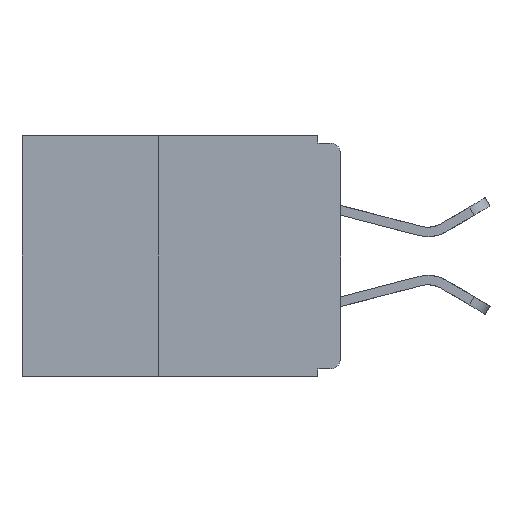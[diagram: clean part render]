
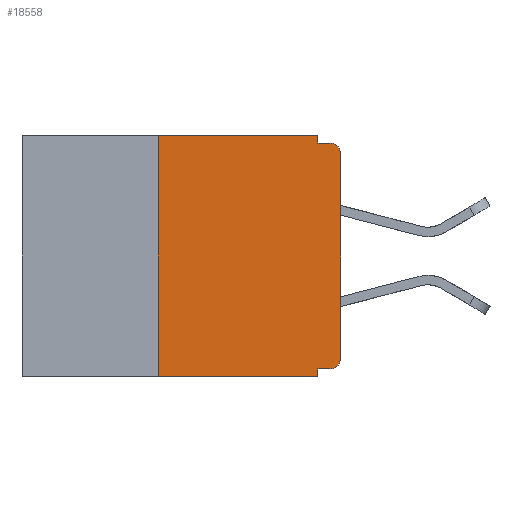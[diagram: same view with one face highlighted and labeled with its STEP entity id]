
A CAD part, left-side view. The second image highlights one B-rep face of the part: STEP entity #18558.
In plain terms, the highlighted planar face has unit normal (-1, 0, 0).
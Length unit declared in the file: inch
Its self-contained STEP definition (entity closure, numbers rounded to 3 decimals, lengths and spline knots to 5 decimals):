
#775 = ORIENTED_EDGE ( 'NONE', *, *, #17930, .F. ) ;
#1948 = CARTESIAN_POINT ( 'NONE',  ( 0., 0.25, -0.33 ) ) ;
#2475 = CARTESIAN_POINT ( 'NONE',  ( 0., 0.015, -0.01 ) ) ;
#2659 = CARTESIAN_POINT ( 'NONE',  ( 0., 0.031, 0. ) ) ;
#2809 = CARTESIAN_POINT ( 'NONE',  ( 0., 0.015, -0.025 ) ) ;
#2883 = DIRECTION ( 'NONE',  ( -1., 0., 0. ) ) ;
#2923 = CIRCLE ( 'NONE', #19588, 0.015 ) ;
#2995 = LINE ( 'NONE', #13170, #19923 ) ;
#3387 = LINE ( 'NONE', #9181, #15979 ) ;
#3621 = DIRECTION ( 'NONE',  ( 0., 0., 1. ) ) ;
#3716 = EDGE_CURVE ( 'NONE', #3820, #6808, #9754, .T. ) ;
#3820 = VERTEX_POINT ( 'NONE', #16730 ) ;
#4018 = CARTESIAN_POINT ( 'NONE',  ( 0., 0.437, -0.33 ) ) ;
#4341 = VECTOR ( 'NONE', #11575, 39.37008 ) ;
#4494 = DIRECTION ( 'NONE',  ( 0., 0., -1. ) ) ;
#4537 = VERTEX_POINT ( 'NONE', #20589 ) ;
#4973 = CIRCLE ( 'NONE', #15085, 0.015 ) ;
#4975 = VERTEX_POINT ( 'NONE', #13607 ) ;
#5214 = VERTEX_POINT ( 'NONE', #2659 ) ;
#5506 = AXIS2_PLACEMENT_3D ( 'NONE', #8097, #12951, #21109 ) ;
#5815 = VERTEX_POINT ( 'NONE', #5926 ) ;
#5926 = CARTESIAN_POINT ( 'NONE',  ( 0., 0.25, 0. ) ) ;
#6296 = EDGE_LOOP ( 'NONE', ( #6617, #12294, #13657, #19914, #775, #10690, #9777, #7531, #16128, #19337 ) ) ;
#6616 = CARTESIAN_POINT ( 'NONE',  ( 0., 0.015, -0.32 ) ) ;
#6617 = ORIENTED_EDGE ( 'NONE', *, *, #21088, .T. ) ;
#6808 = VERTEX_POINT ( 'NONE', #11500 ) ;
#7531 = ORIENTED_EDGE ( 'NONE', *, *, #3716, .F. ) ;
#7636 = LINE ( 'NONE', #16426, #20148 ) ;
#8097 = CARTESIAN_POINT ( 'NONE',  ( 0., 0.437, 0. ) ) ;
#8129 = DIRECTION ( 'NONE',  ( 0., -1., 0. ) ) ;
#8665 = VERTEX_POINT ( 'NONE', #13303 ) ;
#8786 = EDGE_CURVE ( 'NONE', #5214, #15198, #13096, .T. ) ;
#9181 = CARTESIAN_POINT ( 'NONE',  ( 0., 0., -0.01 ) ) ;
#9744 = PLANE ( 'NONE',  #5506 ) ;
#9754 = LINE ( 'NONE', #9954, #4341 ) ;
#9777 = ORIENTED_EDGE ( 'NONE', *, *, #13470, .T. ) ;
#9954 = CARTESIAN_POINT ( 'NONE',  ( 0., 0.031, -0.33 ) ) ;
#10346 = DIRECTION ( 'NONE',  ( 0., 0., -1. ) ) ;
#10690 = ORIENTED_EDGE ( 'NONE', *, *, #18111, .F. ) ;
#10864 = DIRECTION ( 'NONE',  ( 0., -1., 0. ) ) ;
#11077 = FACE_OUTER_BOUND ( 'NONE', #6296, .T. ) ;
#11475 = VERTEX_POINT ( 'NONE', #2475 ) ;
#11500 = CARTESIAN_POINT ( 'NONE',  ( 0., 0.031, -0.33 ) ) ;
#11575 = DIRECTION ( 'NONE',  ( 0., 0., -1. ) ) ;
#12294 = ORIENTED_EDGE ( 'NONE', *, *, #15626, .T. ) ;
#12762 = CARTESIAN_POINT ( 'NONE',  ( 0., 0.015, -0.305 ) ) ;
#12839 = CARTESIAN_POINT ( 'NONE',  ( 0., 0.031, -0.01 ) ) ;
#12951 = DIRECTION ( 'NONE',  ( 1., 0., 0. ) ) ;
#13096 = LINE ( 'NONE', #15304, #16939 ) ;
#13170 = CARTESIAN_POINT ( 'NONE',  ( 0., 0., -0.32 ) ) ;
#13303 = CARTESIAN_POINT ( 'NONE',  ( 0., 0., -0.305 ) ) ;
#13470 = EDGE_CURVE ( 'NONE', #4975, #6808, #13477, .T. ) ;
#13477 = LINE ( 'NONE', #4018, #17329 ) ;
#13607 = CARTESIAN_POINT ( 'NONE',  ( 0., 0.25, -0.33 ) ) ;
#13657 = ORIENTED_EDGE ( 'NONE', *, *, #14688, .F. ) ;
#13858 = DIRECTION ( 'NONE',  ( 0., -1., 0. ) ) ;
#14144 = EDGE_CURVE ( 'NONE', #15823, #8665, #4973, .T. ) ;
#14331 = DIRECTION ( 'NONE',  ( -1., 0., 0. ) ) ;
#14412 = DIRECTION ( 'NONE',  ( 0., 0., -1. ) ) ;
#14688 = EDGE_CURVE ( 'NONE', #15198, #11475, #3387, .T. ) ;
#14759 = DIRECTION ( 'NONE',  ( 0., 1., 0. ) ) ;
#15085 = AXIS2_PLACEMENT_3D ( 'NONE', #12762, #2883, #14412 ) ;
#15198 = VERTEX_POINT ( 'NONE', #12839 ) ;
#15225 = LINE ( 'NONE', #19535, #19545 ) ;
#15304 = CARTESIAN_POINT ( 'NONE',  ( 0., 0.031, 0. ) ) ;
#15464 = VECTOR ( 'NONE', #3621, 39.37008 ) ;
#15626 = EDGE_CURVE ( 'NONE', #4537, #11475, #2923, .T. ) ;
#15823 = VERTEX_POINT ( 'NONE', #6616 ) ;
#15979 = VECTOR ( 'NONE', #10864, 39.37008 ) ;
#16128 = ORIENTED_EDGE ( 'NONE', *, *, #20452, .F. ) ;
#16426 = CARTESIAN_POINT ( 'NONE',  ( 0., 0., 0. ) ) ;
#16730 = CARTESIAN_POINT ( 'NONE',  ( 0., 0.031, -0.32 ) ) ;
#16939 = VECTOR ( 'NONE', #10346, 39.37008 ) ;
#17329 = VECTOR ( 'NONE', #13858, 39.37008 ) ;
#17930 = EDGE_CURVE ( 'NONE', #5815, #5214, #15225, .T. ) ;
#18056 = DIRECTION ( 'NONE',  ( 0., 0., 1. ) ) ;
#18111 = EDGE_CURVE ( 'NONE', #4975, #5815, #20278, .T. ) ;
#18558 = ADVANCED_FACE ( 'NONE', ( #11077 ), #9744, .F. ) ;
#19337 = ORIENTED_EDGE ( 'NONE', *, *, #14144, .T. ) ;
#19535 = CARTESIAN_POINT ( 'NONE',  ( 0., 0.437, 0. ) ) ;
#19545 = VECTOR ( 'NONE', #8129, 39.37008 ) ;
#19588 = AXIS2_PLACEMENT_3D ( 'NONE', #2809, #14331, #4494 ) ;
#19914 = ORIENTED_EDGE ( 'NONE', *, *, #8786, .F. ) ;
#19923 = VECTOR ( 'NONE', #14759, 39.37008 ) ;
#20148 = VECTOR ( 'NONE', #18056, 39.37008 ) ;
#20278 = LINE ( 'NONE', #1948, #15464 ) ;
#20452 = EDGE_CURVE ( 'NONE', #15823, #3820, #2995, .T. ) ;
#20589 = CARTESIAN_POINT ( 'NONE',  ( 0., 0., -0.025 ) ) ;
#21088 = EDGE_CURVE ( 'NONE', #8665, #4537, #7636, .T. ) ;
#21109 = DIRECTION ( 'NONE',  ( 0., 0., -1. ) ) ;
